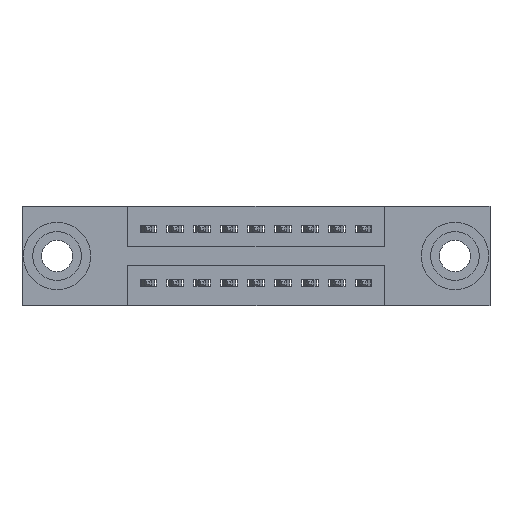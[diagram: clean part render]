
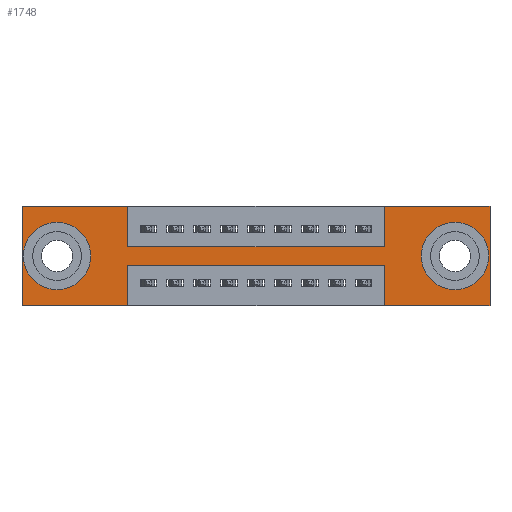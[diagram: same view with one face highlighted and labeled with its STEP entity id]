
A CAD part, front view. The second image highlights one B-rep face of the part: STEP entity #1748.
In plain terms, the highlighted planar face has unit normal (0, -1, 0).
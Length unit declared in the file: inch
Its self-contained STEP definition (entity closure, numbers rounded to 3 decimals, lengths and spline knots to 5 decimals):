
#126 = DIRECTION ( 'NONE',  ( 1., 0., 0. ) ) ;
#155 = DIRECTION ( 'NONE',  ( 0., 0., -1. ) ) ;
#187 = VERTEX_POINT ( 'NONE', #3395 ) ;
#272 = CARTESIAN_POINT ( 'NONE',  ( 0., 0., -0.37 ) ) ;
#455 = EDGE_CURVE ( 'NONE', #4557, #10045, #11844, .T. ) ;
#520 = EDGE_CURVE ( 'NONE', #7839, #11882, #4342, .T. ) ;
#612 = ORIENTED_EDGE ( 'NONE', *, *, #5244, .T. ) ;
#625 = ORIENTED_EDGE ( 'NONE', *, *, #5791, .T. ) ;
#665 = ORIENTED_EDGE ( 'NONE', *, *, #7978, .T. ) ;
#696 = ORIENTED_EDGE ( 'NONE', *, *, #520, .T. ) ;
#740 = ORIENTED_EDGE ( 'NONE', *, *, #7584, .F. ) ;
#757 = DIRECTION ( 'NONE',  ( 0., 1., 0. ) ) ;
#777 = ORIENTED_EDGE ( 'NONE', *, *, #7884, .F. ) ;
#885 = DIRECTION ( 'NONE',  ( 0., 0., -1. ) ) ;
#908 = CARTESIAN_POINT ( 'NONE',  ( 0.3925, 0., 0. ) ) ;
#928 = PLANE ( 'NONE',  #5882 ) ;
#1004 = CARTESIAN_POINT ( 'NONE',  ( 0., 0., -0.37 ) ) ;
#1029 = DIRECTION ( 'NONE',  ( 0., 1., 0. ) ) ;
#1043 = VECTOR ( 'NONE', #5665, 39.37008 ) ;
#1106 = ORIENTED_EDGE ( 'NONE', *, *, #8262, .F. ) ;
#1109 = DIRECTION ( 'NONE',  ( 0., -1., 0. ) ) ;
#1208 = CIRCLE ( 'NONE', #7171, 0.078 ) ;
#1321 = EDGE_CURVE ( 'NONE', #3193, #4557, #5985, .T. ) ;
#1493 = ORIENTED_EDGE ( 'NONE', *, *, #8713, .F. ) ;
#1577 = CARTESIAN_POINT ( 'NONE',  ( 0.13, 0., -0.263 ) ) ;
#1748 = ADVANCED_FACE ( 'NONE', ( #4177, #3880, #6684 ), #928, .T. ) ;
#1976 = VECTOR ( 'NONE', #6020, 39.37008 ) ;
#2279 = CARTESIAN_POINT ( 'NONE',  ( 0.3925, 0., -0.15 ) ) ;
#2334 = DIRECTION ( 'NONE',  ( 0., 0., -1. ) ) ;
#2410 = ORIENTED_EDGE ( 'NONE', *, *, #455, .F. ) ;
#2632 = CARTESIAN_POINT ( 'NONE',  ( 0.3925, 0., 0. ) ) ;
#2867 = CARTESIAN_POINT ( 'NONE',  ( 0., 0., 0. ) ) ;
#2911 = DIRECTION ( 'NONE',  ( 1., 0., 0. ) ) ;
#3193 = VERTEX_POINT ( 'NONE', #8841 ) ;
#3200 = CARTESIAN_POINT ( 'NONE',  ( 0., 0., 0. ) ) ;
#3214 = CARTESIAN_POINT ( 'NONE',  ( 0.3925, 0., -0.15 ) ) ;
#3289 = CARTESIAN_POINT ( 'NONE',  ( 1.3425, 0., -0.37 ) ) ;
#3373 = CARTESIAN_POINT ( 'NONE',  ( 1.3425, 0., 0. ) ) ;
#3381 = VERTEX_POINT ( 'NONE', #11314 ) ;
#3395 = CARTESIAN_POINT ( 'NONE',  ( 1.605, 0., -0.107 ) ) ;
#3665 = DIRECTION ( 'NONE',  ( -1., 0., 0. ) ) ;
#3840 = VECTOR ( 'NONE', #7030, 39.37008 ) ;
#3880 = FACE_BOUND ( 'NONE', #12136, .T. ) ;
#3919 = EDGE_CURVE ( 'NONE', #9434, #4529, #9796, .T. ) ;
#3931 = CARTESIAN_POINT ( 'NONE',  ( 1.3425, 0., 0. ) ) ;
#4137 = LINE ( 'NONE', #9678, #3840 ) ;
#4177 = FACE_BOUND ( 'NONE', #4783, .T. ) ;
#4209 = LINE ( 'NONE', #3214, #8828 ) ;
#4236 = DIRECTION ( 'NONE',  ( 0., 0., 1. ) ) ;
#4342 = CIRCLE ( 'NONE', #8661, 0.078 ) ;
#4386 = ORIENTED_EDGE ( 'NONE', *, *, #11756, .F. ) ;
#4421 = ORIENTED_EDGE ( 'NONE', *, *, #3919, .F. ) ;
#4504 = CIRCLE ( 'NONE', #8240, 0.078 ) ;
#4529 = VERTEX_POINT ( 'NONE', #2279 ) ;
#4557 = VERTEX_POINT ( 'NONE', #7085 ) ;
#4579 = LINE ( 'NONE', #8710, #1976 ) ;
#4783 = EDGE_LOOP ( 'NONE', ( #612, #625 ) ) ;
#4796 = CARTESIAN_POINT ( 'NONE',  ( 0., 0., -0.37 ) ) ;
#4960 = VECTOR ( 'NONE', #11684, 39.37008 ) ;
#5002 = EDGE_LOOP ( 'NONE', ( #740, #777, #1106, #2410, #8554, #1493, #12117, #4386, #4421, #5063, #8486, #9858 ) ) ;
#5063 = ORIENTED_EDGE ( 'NONE', *, *, #5135, .F. ) ;
#5135 = EDGE_CURVE ( 'NONE', #7121, #9434, #5729, .T. ) ;
#5244 = EDGE_CURVE ( 'NONE', #187, #7061, #4504, .T. ) ;
#5428 = VECTOR ( 'NONE', #11281, 39.37008 ) ;
#5665 = DIRECTION ( 'NONE',  ( 0., 0., -1. ) ) ;
#5729 = LINE ( 'NONE', #8662, #5428 ) ;
#5765 = CARTESIAN_POINT ( 'NONE',  ( 1.735, 0., 0. ) ) ;
#5791 = EDGE_CURVE ( 'NONE', #7061, #187, #1208, .T. ) ;
#5882 = AXIS2_PLACEMENT_3D ( 'NONE', #1004, #1109, #885 ) ;
#5985 = LINE ( 'NONE', #5765, #1043 ) ;
#6020 = DIRECTION ( 'NONE',  ( 0., 0., 1. ) ) ;
#6090 = LINE ( 'NONE', #3373, #9985 ) ;
#6127 = DIRECTION ( 'NONE',  ( 0., 1., 0. ) ) ;
#6217 = VERTEX_POINT ( 'NONE', #9166 ) ;
#6219 = DIRECTION ( 'NONE',  ( -1., 0., 0. ) ) ;
#6315 = CARTESIAN_POINT ( 'NONE',  ( 1.3425, 0., -0.15 ) ) ;
#6446 = AXIS2_PLACEMENT_3D ( 'NONE', #6629, #757, #7521 ) ;
#6514 = CARTESIAN_POINT ( 'NONE',  ( 0.3925, 0., -0.22 ) ) ;
#6629 = CARTESIAN_POINT ( 'NONE',  ( 0.13, 0., -0.185 ) ) ;
#6684 = FACE_OUTER_BOUND ( 'NONE', #5002, .T. ) ;
#6772 = LINE ( 'NONE', #3289, #11195 ) ;
#6864 = CARTESIAN_POINT ( 'NONE',  ( 1.3425, 0., -0.37 ) ) ;
#6867 = CARTESIAN_POINT ( 'NONE',  ( 1.605, 0., -0.185 ) ) ;
#6920 = VECTOR ( 'NONE', #2911, 39.37008 ) ;
#7030 = DIRECTION ( 'NONE',  ( 0., 0., -1. ) ) ;
#7061 = VERTEX_POINT ( 'NONE', #9534 ) ;
#7085 = CARTESIAN_POINT ( 'NONE',  ( 1.735, 0., -0.37 ) ) ;
#7121 = VERTEX_POINT ( 'NONE', #3200 ) ;
#7171 = AXIS2_PLACEMENT_3D ( 'NONE', #6867, #1029, #7766 ) ;
#7436 = VECTOR ( 'NONE', #2334, 39.37008 ) ;
#7521 = DIRECTION ( 'NONE',  ( 0., 0., 1. ) ) ;
#7584 = EDGE_CURVE ( 'NONE', #7991, #6217, #4137, .T. ) ;
#7691 = EDGE_CURVE ( 'NONE', #11232, #8778, #6090, .T. ) ;
#7766 = DIRECTION ( 'NONE',  ( 0., 0., -1. ) ) ;
#7839 = VERTEX_POINT ( 'NONE', #1577 ) ;
#7884 = EDGE_CURVE ( 'NONE', #3381, #7991, #8333, .T. ) ;
#7978 = EDGE_CURVE ( 'NONE', #11882, #7839, #9570, .T. ) ;
#7991 = VERTEX_POINT ( 'NONE', #11950 ) ;
#8240 = AXIS2_PLACEMENT_3D ( 'NONE', #11461, #6127, #155 ) ;
#8262 = EDGE_CURVE ( 'NONE', #10045, #3381, #6772, .T. ) ;
#8333 = LINE ( 'NONE', #6514, #10657 ) ;
#8342 = EDGE_CURVE ( 'NONE', #6217, #9913, #10924, .T. ) ;
#8486 = ORIENTED_EDGE ( 'NONE', *, *, #8922, .F. ) ;
#8554 = ORIENTED_EDGE ( 'NONE', *, *, #1321, .F. ) ;
#8661 = AXIS2_PLACEMENT_3D ( 'NONE', #11135, #11122, #11110 ) ;
#8662 = CARTESIAN_POINT ( 'NONE',  ( 0., 0., 0. ) ) ;
#8710 = CARTESIAN_POINT ( 'NONE',  ( 0., 0., 0. ) ) ;
#8713 = EDGE_CURVE ( 'NONE', #8778, #3193, #9572, .T. ) ;
#8778 = VERTEX_POINT ( 'NONE', #3931 ) ;
#8828 = VECTOR ( 'NONE', #126, 39.37008 ) ;
#8841 = CARTESIAN_POINT ( 'NONE',  ( 1.735, 0., 0. ) ) ;
#8922 = EDGE_CURVE ( 'NONE', #9913, #7121, #4579, .T. ) ;
#9166 = CARTESIAN_POINT ( 'NONE',  ( 0.3925, 0., -0.37 ) ) ;
#9434 = VERTEX_POINT ( 'NONE', #908 ) ;
#9534 = CARTESIAN_POINT ( 'NONE',  ( 1.605, 0., -0.263 ) ) ;
#9570 = CIRCLE ( 'NONE', #6446, 0.078 ) ;
#9572 = LINE ( 'NONE', #2867, #6920 ) ;
#9678 = CARTESIAN_POINT ( 'NONE',  ( 0.3925, 0., -0.37 ) ) ;
#9796 = LINE ( 'NONE', #2632, #7436 ) ;
#9858 = ORIENTED_EDGE ( 'NONE', *, *, #8342, .F. ) ;
#9913 = VERTEX_POINT ( 'NONE', #4796 ) ;
#9985 = VECTOR ( 'NONE', #10658, 39.37008 ) ;
#10045 = VERTEX_POINT ( 'NONE', #6864 ) ;
#10649 = VECTOR ( 'NONE', #6219, 39.37008 ) ;
#10657 = VECTOR ( 'NONE', #3665, 39.37008 ) ;
#10658 = DIRECTION ( 'NONE',  ( 0., 0., 1. ) ) ;
#10924 = LINE ( 'NONE', #272, #10649 ) ;
#11110 = DIRECTION ( 'NONE',  ( 0., 0., 1. ) ) ;
#11122 = DIRECTION ( 'NONE',  ( 0., 1., 0. ) ) ;
#11135 = CARTESIAN_POINT ( 'NONE',  ( 0.13, 0., -0.185 ) ) ;
#11195 = VECTOR ( 'NONE', #4236, 39.37008 ) ;
#11232 = VERTEX_POINT ( 'NONE', #6315 ) ;
#11281 = DIRECTION ( 'NONE',  ( 1., 0., 0. ) ) ;
#11314 = CARTESIAN_POINT ( 'NONE',  ( 1.3425, 0., -0.22 ) ) ;
#11461 = CARTESIAN_POINT ( 'NONE',  ( 1.605, 0., -0.185 ) ) ;
#11593 = CARTESIAN_POINT ( 'NONE',  ( 0.13, 0., -0.107 ) ) ;
#11684 = DIRECTION ( 'NONE',  ( -1., 0., 0. ) ) ;
#11700 = CARTESIAN_POINT ( 'NONE',  ( 0., 0., -0.37 ) ) ;
#11756 = EDGE_CURVE ( 'NONE', #4529, #11232, #4209, .T. ) ;
#11844 = LINE ( 'NONE', #11700, #4960 ) ;
#11882 = VERTEX_POINT ( 'NONE', #11593 ) ;
#11950 = CARTESIAN_POINT ( 'NONE',  ( 0.3925, 0., -0.22 ) ) ;
#12117 = ORIENTED_EDGE ( 'NONE', *, *, #7691, .F. ) ;
#12136 = EDGE_LOOP ( 'NONE', ( #665, #696 ) ) ;
